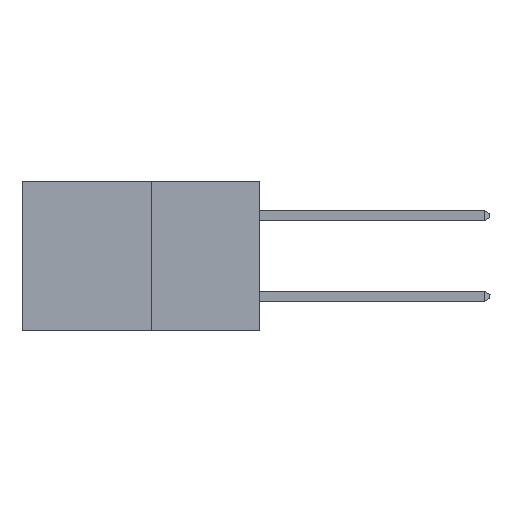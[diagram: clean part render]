
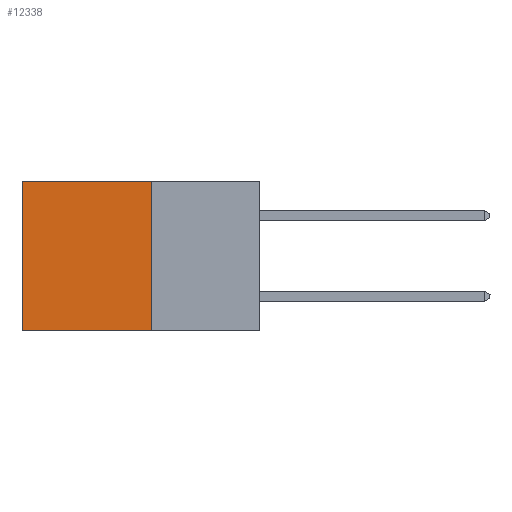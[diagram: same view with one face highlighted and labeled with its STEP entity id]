
A CAD part, left-side view. The second image highlights one B-rep face of the part: STEP entity #12338.
In plain terms, the highlighted planar face has unit normal (-1, 0, 0).
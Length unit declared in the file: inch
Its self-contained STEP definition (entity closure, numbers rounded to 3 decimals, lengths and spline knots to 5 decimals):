
#307 = VECTOR ( 'NONE', #7968, 39.37008 ) ;
#416 = CARTESIAN_POINT ( 'NONE',  ( 0.277, 0.27, -0.37 ) ) ;
#2340 = VECTOR ( 'NONE', #13605, 39.37008 ) ;
#2627 = CARTESIAN_POINT ( 'NONE',  ( 0.277, 0.59, 0. ) ) ;
#2774 = CARTESIAN_POINT ( 'NONE',  ( 0.277, 0.27, 0. ) ) ;
#3266 = VECTOR ( 'NONE', #21731, 39.37008 ) ;
#3301 = CARTESIAN_POINT ( 'NONE',  ( 0.277, 0.27, 0. ) ) ;
#3599 = CARTESIAN_POINT ( 'NONE',  ( 0.277, 0.27, -0.37 ) ) ;
#5493 = EDGE_CURVE ( 'NONE', #23068, #16497, #20505, .T. ) ;
#6607 = CARTESIAN_POINT ( 'NONE',  ( 0.277, 0.59, -0.37 ) ) ;
#7429 = EDGE_CURVE ( 'NONE', #12916, #15340, #13186, .T. ) ;
#7968 = DIRECTION ( 'NONE',  ( 0., 0., -1. ) ) ;
#7984 = FACE_OUTER_BOUND ( 'NONE', #18806, .T. ) ;
#8141 = CARTESIAN_POINT ( 'NONE',  ( 0.277, 0.27, -0.37 ) ) ;
#8618 = DIRECTION ( 'NONE',  ( 1., 0., 0. ) ) ;
#12338 = ADVANCED_FACE ( 'NONE', ( #7984 ), #14186, .F. ) ;
#12916 = VERTEX_POINT ( 'NONE', #2627 ) ;
#13186 = LINE ( 'NONE', #6607, #3266 ) ;
#13250 = CARTESIAN_POINT ( 'NONE',  ( 0.277, 0.59, -0.37 ) ) ;
#13605 = DIRECTION ( 'NONE',  ( 0., 1., 0. ) ) ;
#14186 = PLANE ( 'NONE',  #17048 ) ;
#14238 = EDGE_CURVE ( 'NONE', #16497, #15340, #21241, .T. ) ;
#15340 = VERTEX_POINT ( 'NONE', #13250 ) ;
#16421 = DIRECTION ( 'NONE',  ( 0., 1., 0. ) ) ;
#16497 = VERTEX_POINT ( 'NONE', #3599 ) ;
#17048 = AXIS2_PLACEMENT_3D ( 'NONE', #18035, #8618, #21873 ) ;
#17628 = ORIENTED_EDGE ( 'NONE', *, *, #5493, .F. ) ;
#18035 = CARTESIAN_POINT ( 'NONE',  ( 0.277, 0.27, -0.37 ) ) ;
#18806 = EDGE_LOOP ( 'NONE', ( #21296, #20546, #17628, #24027 ) ) ;
#18839 = VECTOR ( 'NONE', #16421, 39.37008 ) ;
#19173 = EDGE_CURVE ( 'NONE', #23068, #12916, #19454, .T. ) ;
#19454 = LINE ( 'NONE', #3301, #18839 ) ;
#20505 = LINE ( 'NONE', #8141, #307 ) ;
#20546 = ORIENTED_EDGE ( 'NONE', *, *, #14238, .F. ) ;
#21241 = LINE ( 'NONE', #416, #2340 ) ;
#21296 = ORIENTED_EDGE ( 'NONE', *, *, #7429, .T. ) ;
#21731 = DIRECTION ( 'NONE',  ( 0., 0., -1. ) ) ;
#21873 = DIRECTION ( 'NONE',  ( 0., 0., -1. ) ) ;
#23068 = VERTEX_POINT ( 'NONE', #2774 ) ;
#24027 = ORIENTED_EDGE ( 'NONE', *, *, #19173, .T. ) ;
